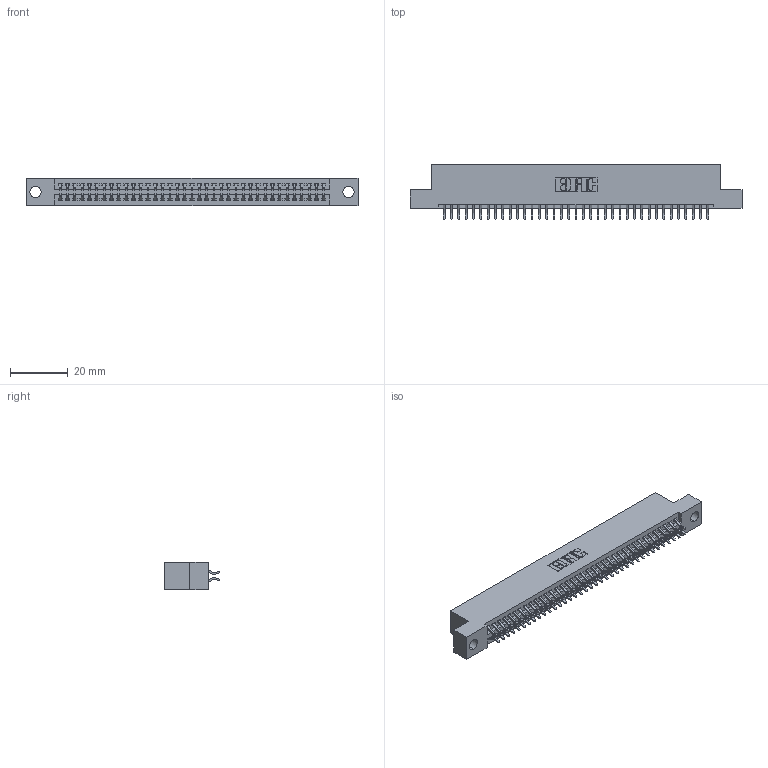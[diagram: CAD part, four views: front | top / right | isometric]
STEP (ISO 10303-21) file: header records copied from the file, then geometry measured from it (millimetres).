
FILE_DESCRIPTION (( 'STEP AP203' ), '1' );
FILE_NAME ('345-074-556-204.STEP', '2018-10-02T13:29:57', ( '' ), ( '' ), 'SwSTEP 2.0', 'SolidWorks 2016', '' );
FILE_SCHEMA (( 'CONFIG_CONTROL_DESIGN' ));
Length unit declared in the file: inch
Products named in the file (3): 345-074-556-204; 345 Part_Flush Mounting Lugs - 0.156 Dia-TH; 345-292-001_556 Tail
Assembly tree (75 placements, depth 2):
  345-074-556-204
    345 Part_Flush Mounting Lugs - 0.156 Dia-TH
    345-292-001_556 Tail  x74
Bounding box: 115.19 x 19.24 x 9.4 mm (x, y, z)
Volume: 11052.4 mm3; surface area: 15990.8 mm2
Topology: 75 solids, 75 shells, 4270 faces, 12699 edges, 8366 vertices
Faces by surface type: plane 2818, cylinder 1452
Entity records: 29927 total; most frequent: CARTESIAN_POINT 5036, ORIENTED_EDGE 4958, DIRECTION 4435, EDGE_CURVE 2479, VECTOR 2191, LINE 2191, VERTEX_POINT 1650, AXIS2_PLACEMENT_3D 1122
